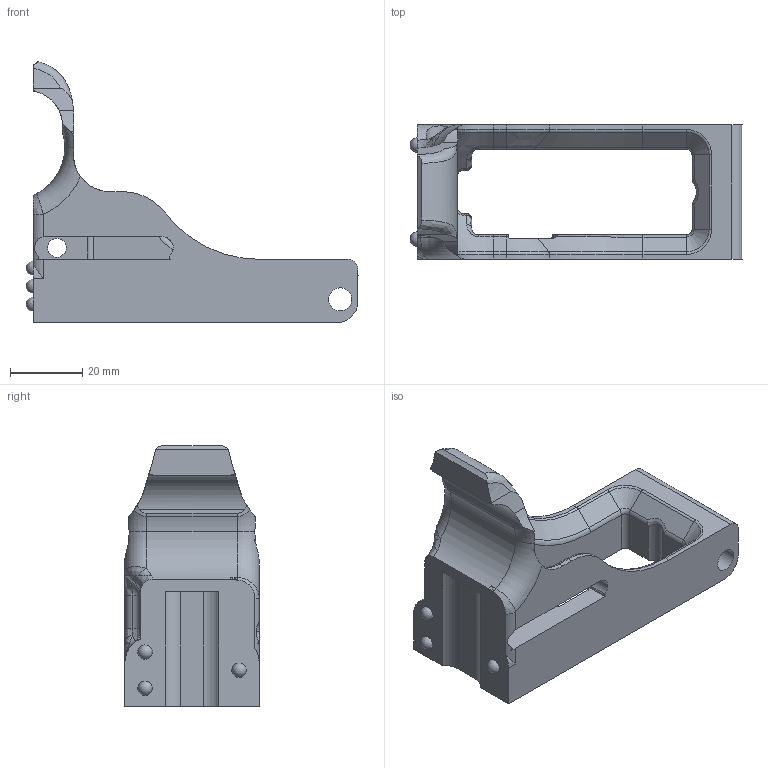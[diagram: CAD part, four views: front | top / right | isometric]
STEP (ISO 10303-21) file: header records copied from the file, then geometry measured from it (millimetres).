
FILE_DESCRIPTION (( 'STEP AP214' ), '1' );
FILE_NAME ('Magwell_3c.STEP', '2015-10-23T19:49:56', ( 'WarFairy' ), ( '' ), 'SwSTEP 2.0', 'SolidWorks 2015', '' );
FILE_SCHEMA (( 'AUTOMOTIVE_DESIGN' ));
Length unit declared in the file: millimetre
Products named in the file (1): Magwell_3c
Bounding box: 91.82 x 37.13 x 72.14 mm (x, y, z)
Volume: 42204.4 mm3; surface area: 18455 mm2
Topology: 1 solids, 3 shells, 221 faces, 608 edges, 383 vertices
Faces by surface type: cylinder 77, plane 60, bspline 45, torus 28, cone 8, sphere 3
Entity records: 9319 total; most frequent: CARTESIAN_POINT 4108, ORIENTED_EDGE 1182, DIRECTION 971, EDGE_CURVE 591, VERTEX_POINT 377, AXIS2_PLACEMENT_3D 372, EDGE_LOOP 232, VECTOR 227
